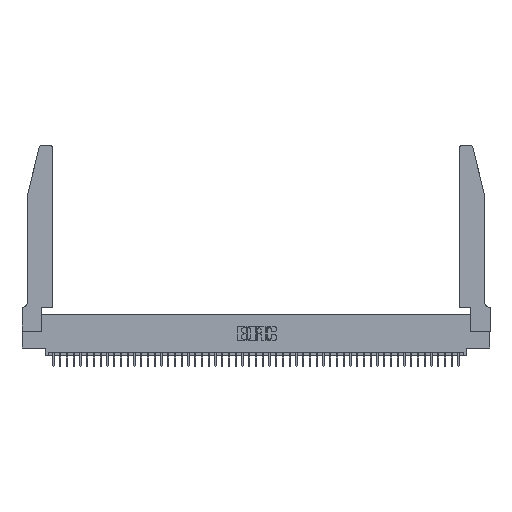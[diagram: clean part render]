
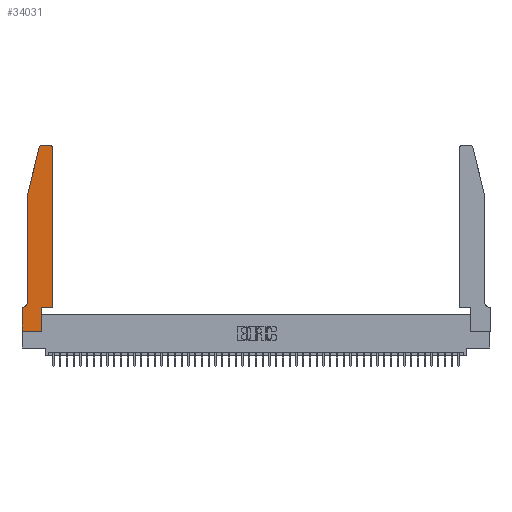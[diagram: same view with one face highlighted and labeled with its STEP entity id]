
A CAD part, top view. The second image highlights one B-rep face of the part: STEP entity #34031.
In plain terms, the highlighted planar face has unit normal (0, 0, 1).
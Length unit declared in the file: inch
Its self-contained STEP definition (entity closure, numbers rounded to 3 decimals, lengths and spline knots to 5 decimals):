
#785 = EDGE_CURVE ( 'NONE', #19338, #44165, #19299, .T. ) ;
#1261 = DIRECTION ( 'NONE',  ( 0., 0., 1. ) ) ;
#1365 = CARTESIAN_POINT ( 'NONE',  ( 0.4505, 2.72, 0.37 ) ) ;
#1639 = CARTESIAN_POINT ( 'NONE',  ( 0., 0.35, 0.37 ) ) ;
#1937 = CARTESIAN_POINT ( 'NONE',  ( 0.284, 2.72, 0.37 ) ) ;
#1950 = VERTEX_POINT ( 'NONE', #4415 ) ;
#2243 = CARTESIAN_POINT ( 'NONE',  ( 0.0755, 0.42, 0.37 ) ) ;
#2803 = ORIENTED_EDGE ( 'NONE', *, *, #19549, .T. ) ;
#2879 = LINE ( 'NONE', #35660, #44248 ) ;
#3683 = DIRECTION ( 'NONE',  ( -1., 0., 0. ) ) ;
#4415 = CARTESIAN_POINT ( 'NONE',  ( 0.25487, 2.72718, 0.37 ) ) ;
#4458 = VERTEX_POINT ( 'NONE', #16447 ) ;
#4869 = LINE ( 'NONE', #24628, #24444 ) ;
#5596 = DIRECTION ( 'NONE',  ( 1., 0., 0. ) ) ;
#5905 = DIRECTION ( 'NONE',  ( 1., 0., 0. ) ) ;
#6320 = CARTESIAN_POINT ( 'NONE',  ( 0.2865, 0., 0.37 ) ) ;
#6470 = EDGE_CURVE ( 'NONE', #44165, #20994, #4869, .T. ) ;
#6729 = EDGE_LOOP ( 'NONE', ( #37082, #10104, #20402, #2803, #43653, #48637, #22977, #47422, #19659, #8475, #16599, #24370 ) ) ;
#7083 = CARTESIAN_POINT ( 'NONE',  ( 0., 0., 0.37 ) ) ;
#7219 = DIRECTION ( 'NONE',  ( 1., 0., 0. ) ) ;
#7773 = CIRCLE ( 'NONE', #23972, 0.07 ) ;
#8475 = ORIENTED_EDGE ( 'NONE', *, *, #35002, .T. ) ;
#8690 = CARTESIAN_POINT ( 'NONE',  ( 0., 0., 0.37 ) ) ;
#9258 = CARTESIAN_POINT ( 'NONE',  ( 0.0755, 2., 0.37 ) ) ;
#10104 = ORIENTED_EDGE ( 'NONE', *, *, #47458, .T. ) ;
#10105 = EDGE_CURVE ( 'NONE', #42003, #17815, #23526, .T. ) ;
#10196 = CARTESIAN_POINT ( 'NONE',  ( 0.4505, 0.35, 0.37 ) ) ;
#11513 = LINE ( 'NONE', #49743, #42478 ) ;
#12240 = CIRCLE ( 'NONE', #26023, 0.03 ) ;
#12796 = DIRECTION ( 'NONE',  ( 1., 0., 0. ) ) ;
#12852 = FACE_OUTER_BOUND ( 'NONE', #6729, .T. ) ;
#14908 = LINE ( 'NONE', #9258, #36028 ) ;
#16447 = CARTESIAN_POINT ( 'NONE',  ( 0.0755, 2., 0.37 ) ) ;
#16599 = ORIENTED_EDGE ( 'NONE', *, *, #46613, .T. ) ;
#16969 = DIRECTION ( 'NONE',  ( -1., 0., 0. ) ) ;
#17815 = VERTEX_POINT ( 'NONE', #27035 ) ;
#18013 = CARTESIAN_POINT ( 'NONE',  ( 0.4205, 2.75, 0.37 ) ) ;
#18332 = CARTESIAN_POINT ( 'NONE',  ( 0.0755, 2., 0.37 ) ) ;
#19057 = VECTOR ( 'NONE', #36228, 39.37008 ) ;
#19266 = LINE ( 'NONE', #18332, #38612 ) ;
#19299 = CIRCLE ( 'NONE', #22731, 0.03 ) ;
#19338 = VERTEX_POINT ( 'NONE', #1365 ) ;
#19549 = EDGE_CURVE ( 'NONE', #4458, #29606, #19266, .T. ) ;
#19659 = ORIENTED_EDGE ( 'NONE', *, *, #48773, .T. ) ;
#20402 = ORIENTED_EDGE ( 'NONE', *, *, #42356, .T. ) ;
#20489 = DIRECTION ( 'NONE',  ( 0., 0., -1. ) ) ;
#20994 = VERTEX_POINT ( 'NONE', #34243 ) ;
#22254 = DIRECTION ( 'NONE',  ( 0., -1., 0. ) ) ;
#22731 = AXIS2_PLACEMENT_3D ( 'NONE', #24726, #1261, #28595 ) ;
#22977 = ORIENTED_EDGE ( 'NONE', *, *, #10105, .T. ) ;
#23526 = LINE ( 'NONE', #7083, #44091 ) ;
#23927 = VERTEX_POINT ( 'NONE', #39577 ) ;
#23934 = EDGE_CURVE ( 'NONE', #29606, #24457, #7773, .T. ) ;
#23972 = AXIS2_PLACEMENT_3D ( 'NONE', #43650, #20489, #47507 ) ;
#24190 = VERTEX_POINT ( 'NONE', #10196 ) ;
#24370 = ORIENTED_EDGE ( 'NONE', *, *, #785, .T. ) ;
#24444 = VECTOR ( 'NONE', #16969, 39.37008 ) ;
#24457 = VERTEX_POINT ( 'NONE', #27218 ) ;
#24628 = CARTESIAN_POINT ( 'NONE',  ( 0.2605, 2.75, 0.37 ) ) ;
#24726 = CARTESIAN_POINT ( 'NONE',  ( 0.4205, 2.72, 0.37 ) ) ;
#25814 = LINE ( 'NONE', #50162, #34833 ) ;
#26023 = AXIS2_PLACEMENT_3D ( 'NONE', #1937, #29233, #5905 ) ;
#27035 = CARTESIAN_POINT ( 'NONE',  ( 0., 0., 0.37 ) ) ;
#27218 = CARTESIAN_POINT ( 'NONE',  ( 0.0055, 0.35, 0.37 ) ) ;
#27361 = VERTEX_POINT ( 'NONE', #6320 ) ;
#27363 = LINE ( 'NONE', #8690, #29785 ) ;
#27546 = EDGE_CURVE ( 'NONE', #24457, #42003, #25814, .T. ) ;
#28476 = CARTESIAN_POINT ( 'NONE',  ( 0.4505, 0.35, 0.37 ) ) ;
#28595 = DIRECTION ( 'NONE',  ( 1., 0., 0. ) ) ;
#28932 = DIRECTION ( 'NONE',  ( 0., 0., 1. ) ) ;
#29233 = DIRECTION ( 'NONE',  ( 0., 0., 1. ) ) ;
#29367 = LINE ( 'NONE', #28476, #19057 ) ;
#29606 = VERTEX_POINT ( 'NONE', #2243 ) ;
#29785 = VECTOR ( 'NONE', #12796, 39.37008 ) ;
#30404 = DIRECTION ( 'NONE',  ( 0., -1., 0. ) ) ;
#30730 = EDGE_CURVE ( 'NONE', #17815, #27361, #27363, .T. ) ;
#32577 = DIRECTION ( 'NONE',  ( -0.239, -0.971, 0. ) ) ;
#34031 = ADVANCED_FACE ( 'NONE', ( #12852 ), #44312, .T. ) ;
#34243 = CARTESIAN_POINT ( 'NONE',  ( 0.284, 2.75, 0.37 ) ) ;
#34591 = CARTESIAN_POINT ( 'NONE',  ( 0., 0.35, 0.37 ) ) ;
#34833 = VECTOR ( 'NONE', #3683, 39.37008 ) ;
#35002 = EDGE_CURVE ( 'NONE', #23927, #24190, #11513, .T. ) ;
#35660 = CARTESIAN_POINT ( 'NONE',  ( 0.2865, 0.35, 0.37 ) ) ;
#36028 = VECTOR ( 'NONE', #32577, 39.37008 ) ;
#36228 = DIRECTION ( 'NONE',  ( 0., 1., 0. ) ) ;
#37082 = ORIENTED_EDGE ( 'NONE', *, *, #6470, .T. ) ;
#38612 = VECTOR ( 'NONE', #22254, 39.37008 ) ;
#39559 = DIRECTION ( 'NONE',  ( 0., 1., 0. ) ) ;
#39577 = CARTESIAN_POINT ( 'NONE',  ( 0.2865, 0.35, 0.37 ) ) ;
#42003 = VERTEX_POINT ( 'NONE', #34591 ) ;
#42356 = EDGE_CURVE ( 'NONE', #1950, #4458, #14908, .T. ) ;
#42478 = VECTOR ( 'NONE', #7219, 39.37008 ) ;
#43650 = CARTESIAN_POINT ( 'NONE',  ( 0.0055, 0.42, 0.37 ) ) ;
#43653 = ORIENTED_EDGE ( 'NONE', *, *, #23934, .T. ) ;
#44091 = VECTOR ( 'NONE', #30404, 39.37008 ) ;
#44165 = VERTEX_POINT ( 'NONE', #18013 ) ;
#44248 = VECTOR ( 'NONE', #39559, 39.37008 ) ;
#44312 = PLANE ( 'NONE',  #46348 ) ;
#46348 = AXIS2_PLACEMENT_3D ( 'NONE', #1639, #28932, #5596 ) ;
#46613 = EDGE_CURVE ( 'NONE', #24190, #19338, #29367, .T. ) ;
#47422 = ORIENTED_EDGE ( 'NONE', *, *, #30730, .T. ) ;
#47458 = EDGE_CURVE ( 'NONE', #20994, #1950, #12240, .T. ) ;
#47507 = DIRECTION ( 'NONE',  ( -1., 0., 0. ) ) ;
#48637 = ORIENTED_EDGE ( 'NONE', *, *, #27546, .T. ) ;
#48773 = EDGE_CURVE ( 'NONE', #27361, #23927, #2879, .T. ) ;
#49743 = CARTESIAN_POINT ( 'NONE',  ( 0.4505, 0.35, 0.37 ) ) ;
#50162 = CARTESIAN_POINT ( 'NONE',  ( 0.0755, 0.35, 0.37 ) ) ;
